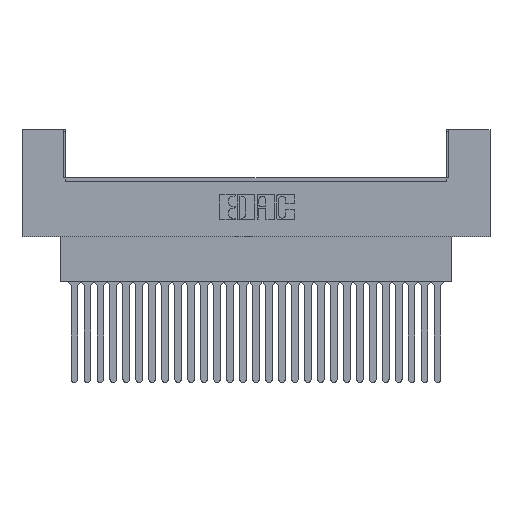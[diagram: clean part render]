
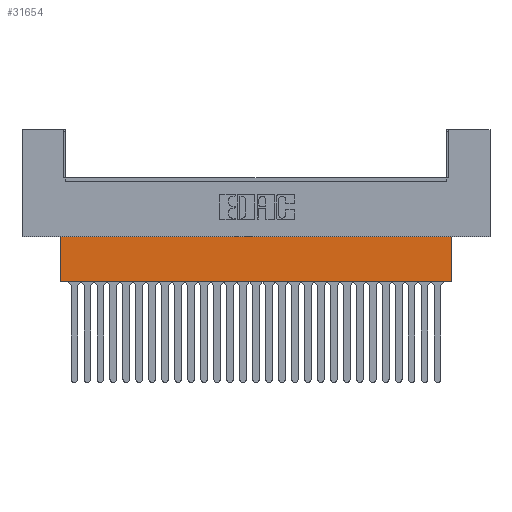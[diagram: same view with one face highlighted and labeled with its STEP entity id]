
A CAD part, top view. The second image highlights one B-rep face of the part: STEP entity #31654.
In plain terms, the highlighted planar face has unit normal (0, 0, 1).
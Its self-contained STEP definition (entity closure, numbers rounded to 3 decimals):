
#1275 = DIRECTION ( 'NONE',  ( 0., 1., 0. ) ) ;
#4334 = VECTOR ( 'NONE', #13200, 1000. ) ;
#4767 = ORIENTED_EDGE ( 'NONE', *, *, #18442, .F. ) ;
#6746 = CARTESIAN_POINT ( 'NONE',  ( 7.468, -8.814, -3.962 ) ) ;
#7169 = AXIS2_PLACEMENT_3D ( 'NONE', #22750, #20482, #1275 ) ;
#7602 = ORIENTED_EDGE ( 'NONE', *, *, #11976, .F. ) ;
#8109 = CARTESIAN_POINT ( 'NONE',  ( 91.592, -8.814, -3.962 ) ) ;
#8477 = ORIENTED_EDGE ( 'NONE', *, *, #12490, .F. ) ;
#9432 = LINE ( 'NONE', #35117, #4334 ) ;
#10509 = DIRECTION ( 'NONE',  ( -1., 0., 0. ) ) ;
#11976 = EDGE_CURVE ( 'NONE', #32911, #25825, #16094, .T. ) ;
#12490 = EDGE_CURVE ( 'NONE', #34912, #32911, #13047, .T. ) ;
#12862 = CARTESIAN_POINT ( 'NONE',  ( 7.468, -8.814, -3.962 ) ) ;
#13047 = LINE ( 'NONE', #8109, #22043 ) ;
#13200 = DIRECTION ( 'NONE',  ( 0., -1., 0. ) ) ;
#13548 = CARTESIAN_POINT ( 'NONE',  ( 7.468, 0., -3.962 ) ) ;
#15877 = CARTESIAN_POINT ( 'NONE',  ( 91.592, 0., -3.962 ) ) ;
#16094 = LINE ( 'NONE', #6746, #25048 ) ;
#17474 = EDGE_LOOP ( 'NONE', ( #8477, #4767, #25930, #7602 ) ) ;
#18442 = EDGE_CURVE ( 'NONE', #20391, #34912, #9432, .T. ) ;
#19392 = DIRECTION ( 'NONE',  ( -1., 0., 0. ) ) ;
#19568 = EDGE_CURVE ( 'NONE', #20391, #25825, #28543, .T. ) ;
#20007 = PLANE ( 'NONE',  #7169 ) ;
#20391 = VERTEX_POINT ( 'NONE', #33120 ) ;
#20482 = DIRECTION ( 'NONE',  ( 0., 0., -1. ) ) ;
#22043 = VECTOR ( 'NONE', #19392, 1000. ) ;
#22750 = CARTESIAN_POINT ( 'NONE',  ( 91.592, 0., -3.962 ) ) ;
#24290 = VECTOR ( 'NONE', #10509, 1000. ) ;
#24573 = CARTESIAN_POINT ( 'NONE',  ( 84.125, -8.814, -3.962 ) ) ;
#25048 = VECTOR ( 'NONE', #25927, 1000. ) ;
#25825 = VERTEX_POINT ( 'NONE', #13548 ) ;
#25927 = DIRECTION ( 'NONE',  ( 0., 1., 0. ) ) ;
#25930 = ORIENTED_EDGE ( 'NONE', *, *, #19568, .T. ) ;
#28543 = LINE ( 'NONE', #15877, #24290 ) ;
#31654 = ADVANCED_FACE ( 'NONE', ( #32329 ), #20007, .F. ) ;
#32329 = FACE_OUTER_BOUND ( 'NONE', #17474, .T. ) ;
#32911 = VERTEX_POINT ( 'NONE', #12862 ) ;
#33120 = CARTESIAN_POINT ( 'NONE',  ( 84.125, 0., -3.962 ) ) ;
#34912 = VERTEX_POINT ( 'NONE', #24573 ) ;
#35117 = CARTESIAN_POINT ( 'NONE',  ( 84.125, -8.814, -3.962 ) ) ;
